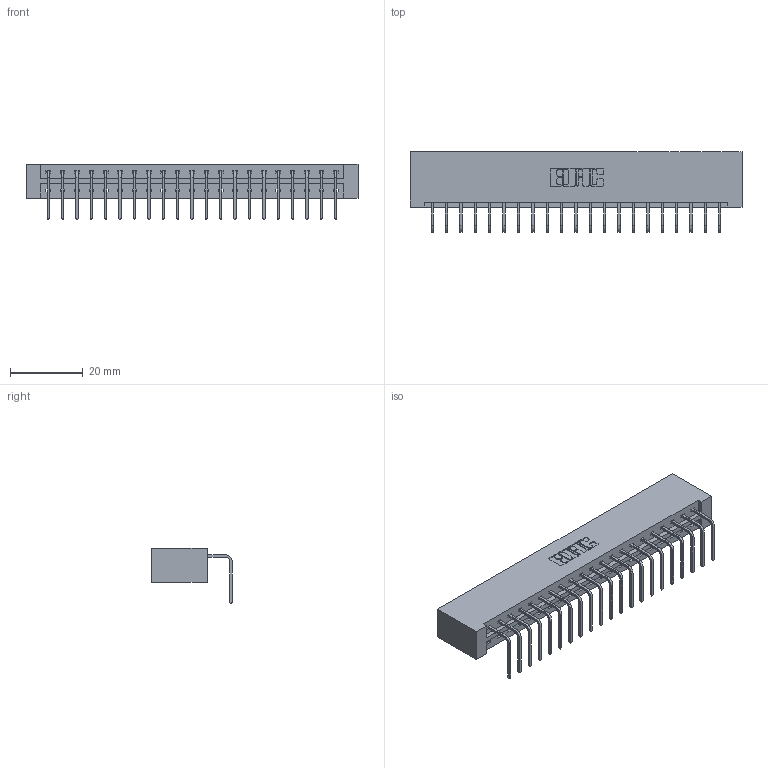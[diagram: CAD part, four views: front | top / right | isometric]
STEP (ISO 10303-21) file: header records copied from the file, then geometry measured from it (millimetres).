
FILE_DESCRIPTION (( 'STEP AP203' ), '1' );
FILE_NAME ('333-021-558-101.STEP', '2018-08-02T01:20:31', ( '' ), ( '' ), 'SwSTEP 2.0', 'SolidWorks 2016', '' );
FILE_SCHEMA (( 'CONFIG_CONTROL_DESIGN' ));
Length unit declared in the file: inch
Products named in the file (3): 333-021-558-101; 333 Part_Lugless; 345-292-001_558 Tail - 2
Assembly tree (22 placements, depth 2):
  333-021-558-101
    333 Part_Lugless
    345-292-001_558 Tail - 2  x21
Bounding box: 91.47 x 22.17 x 15.37 mm (x, y, z)
Volume: 9706.1 mm3; surface area: 10750 mm2
Topology: 22 solids, 22 shells, 1366 faces, 4109 edges, 2710 vertices
Faces by surface type: plane 990, cylinder 376
Entity records: 15361 total; most frequent: CARTESIAN_POINT 2661, ORIENTED_EDGE 2618, DIRECTION 2279, EDGE_CURVE 1309, VECTOR 1189, LINE 1189, VERTEX_POINT 870, AXIS2_PLACEMENT_3D 545
